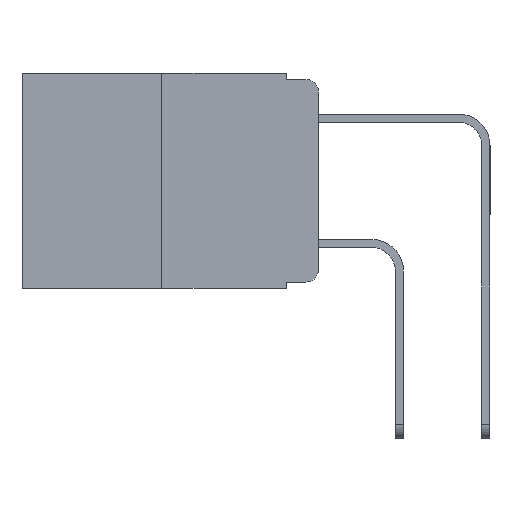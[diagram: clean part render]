
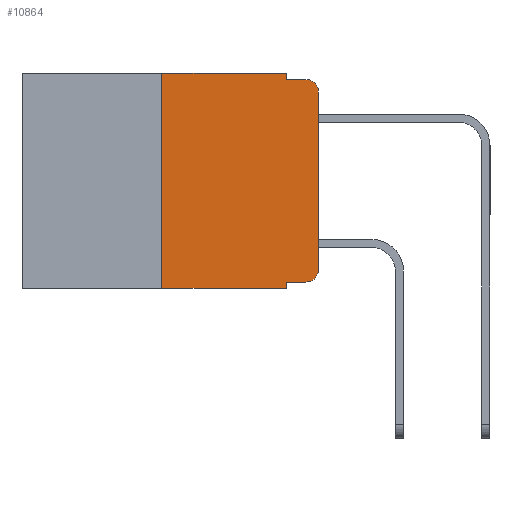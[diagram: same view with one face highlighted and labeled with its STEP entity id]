
A CAD part, left-side view. The second image highlights one B-rep face of the part: STEP entity #10864.
In plain terms, the highlighted planar face has unit normal (-1, 0, 0).
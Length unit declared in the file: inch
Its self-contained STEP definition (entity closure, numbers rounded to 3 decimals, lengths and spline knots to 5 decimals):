
#480 = CARTESIAN_POINT ( 'NONE',  ( 0., 0.051, 0. ) ) ;
#530 = LINE ( 'NONE', #8415, #14699 ) ;
#1100 = DIRECTION ( 'NONE',  ( 0., -1., 0. ) ) ;
#1102 = CIRCLE ( 'NONE', #14284, 0.02 ) ;
#1296 = CARTESIAN_POINT ( 'NONE',  ( 0., 0., 0. ) ) ;
#1386 = VERTEX_POINT ( 'NONE', #8026 ) ;
#1832 = DIRECTION ( 'NONE',  ( -1., 0., 0. ) ) ;
#1882 = DIRECTION ( 'NONE',  ( 0., 0., -1. ) ) ;
#2090 = PLANE ( 'NONE',  #13053 ) ;
#2598 = DIRECTION ( 'NONE',  ( 0., -1., 0. ) ) ;
#2621 = VERTEX_POINT ( 'NONE', #9906 ) ;
#2766 = CARTESIAN_POINT ( 'NONE',  ( 0., 0., -0.313 ) ) ;
#3625 = CARTESIAN_POINT ( 'NONE',  ( 0., 0.473, 0. ) ) ;
#4057 = EDGE_LOOP ( 'NONE', ( #8170, #14215, #16428, #11961, #13609, #15062, #17123, #9033, #10760, #8402 ) ) ;
#4405 = VERTEX_POINT ( 'NONE', #8011 ) ;
#4458 = LINE ( 'NONE', #8059, #11484 ) ;
#4533 = DIRECTION ( 'NONE',  ( 0., 0., 1. ) ) ;
#4945 = DIRECTION ( 'NONE',  ( 0., 0., -1. ) ) ;
#5331 = VERTEX_POINT ( 'NONE', #17863 ) ;
#5490 = CARTESIAN_POINT ( 'NONE',  ( 0., 0.473, 0. ) ) ;
#5586 = EDGE_CURVE ( 'NONE', #4405, #9103, #1102, .T. ) ;
#6154 = LINE ( 'NONE', #11848, #13022 ) ;
#6484 = FACE_OUTER_BOUND ( 'NONE', #4057, .T. ) ;
#6548 = DIRECTION ( 'NONE',  ( 0., 0., -1. ) ) ;
#6557 = EDGE_CURVE ( 'NONE', #1386, #4405, #530, .T. ) ;
#7284 = CARTESIAN_POINT ( 'NONE',  ( 0., 0., -0.03 ) ) ;
#7324 = CARTESIAN_POINT ( 'NONE',  ( 0., 0.051, -0.01 ) ) ;
#7460 = CARTESIAN_POINT ( 'NONE',  ( 0., 0.02, -0.03 ) ) ;
#7497 = EDGE_CURVE ( 'NONE', #1386, #2621, #6154, .T. ) ;
#7759 = VERTEX_POINT ( 'NONE', #15169 ) ;
#8011 = CARTESIAN_POINT ( 'NONE',  ( 0., 0.02, -0.333 ) ) ;
#8026 = CARTESIAN_POINT ( 'NONE',  ( 0., 0.051, -0.333 ) ) ;
#8059 = CARTESIAN_POINT ( 'NONE',  ( 0., 0.051, -0.01 ) ) ;
#8170 = ORIENTED_EDGE ( 'NONE', *, *, #12098, .T. ) ;
#8171 = VECTOR ( 'NONE', #10193, 39.37008 ) ;
#8244 = CIRCLE ( 'NONE', #10957, 0.02 ) ;
#8402 = ORIENTED_EDGE ( 'NONE', *, *, #5586, .T. ) ;
#8415 = CARTESIAN_POINT ( 'NONE',  ( 0., 0.051, -0.333 ) ) ;
#8440 = EDGE_CURVE ( 'NONE', #9852, #5331, #8981, .T. ) ;
#8602 = LINE ( 'NONE', #8787, #8171 ) ;
#8787 = CARTESIAN_POINT ( 'NONE',  ( 0., 0.473, -0.343 ) ) ;
#8847 = DIRECTION ( 'NONE',  ( 0., 0., -1. ) ) ;
#8926 = VERTEX_POINT ( 'NONE', #480 ) ;
#8981 = LINE ( 'NONE', #10157, #12197 ) ;
#9033 = ORIENTED_EDGE ( 'NONE', *, *, #7497, .F. ) ;
#9097 = CARTESIAN_POINT ( 'NONE',  ( 0., 0.051, 0. ) ) ;
#9103 = VERTEX_POINT ( 'NONE', #2766 ) ;
#9157 = VECTOR ( 'NONE', #1882, 39.37008 ) ;
#9165 = VERTEX_POINT ( 'NONE', #7284 ) ;
#9296 = VECTOR ( 'NONE', #11240, 39.37008 ) ;
#9353 = EDGE_CURVE ( 'NONE', #8926, #9755, #9608, .T. ) ;
#9608 = LINE ( 'NONE', #9097, #9157 ) ;
#9755 = VERTEX_POINT ( 'NONE', #7324 ) ;
#9852 = VERTEX_POINT ( 'NONE', #16800 ) ;
#9906 = CARTESIAN_POINT ( 'NONE',  ( 0., 0.051, -0.343 ) ) ;
#9946 = VECTOR ( 'NONE', #2598, 39.37008 ) ;
#10157 = CARTESIAN_POINT ( 'NONE',  ( 0., 0.25, 0. ) ) ;
#10193 = DIRECTION ( 'NONE',  ( 0., -1., 0. ) ) ;
#10279 = EDGE_CURVE ( 'NONE', #9755, #7759, #4458, .T. ) ;
#10437 = CARTESIAN_POINT ( 'NONE',  ( 0., 0.02, -0.313 ) ) ;
#10760 = ORIENTED_EDGE ( 'NONE', *, *, #6557, .T. ) ;
#10864 = ADVANCED_FACE ( 'NONE', ( #6484 ), #2090, .F. ) ;
#10957 = AXIS2_PLACEMENT_3D ( 'NONE', #7460, #16825, #8847 ) ;
#11209 = EDGE_CURVE ( 'NONE', #9165, #7759, #8244, .T. ) ;
#11240 = DIRECTION ( 'NONE',  ( 0., 0., 1. ) ) ;
#11484 = VECTOR ( 'NONE', #17371, 39.37008 ) ;
#11811 = DIRECTION ( 'NONE',  ( 0., 0., -1. ) ) ;
#11848 = CARTESIAN_POINT ( 'NONE',  ( 0., 0.051, 0. ) ) ;
#11961 = ORIENTED_EDGE ( 'NONE', *, *, #9353, .F. ) ;
#12075 = LINE ( 'NONE', #1296, #9296 ) ;
#12098 = EDGE_CURVE ( 'NONE', #9103, #9165, #12075, .T. ) ;
#12197 = VECTOR ( 'NONE', #4533, 39.37008 ) ;
#13022 = VECTOR ( 'NONE', #4945, 39.37008 ) ;
#13053 = AXIS2_PLACEMENT_3D ( 'NONE', #3625, #14660, #6548 ) ;
#13609 = ORIENTED_EDGE ( 'NONE', *, *, #15982, .F. ) ;
#13758 = EDGE_CURVE ( 'NONE', #9852, #2621, #8602, .T. ) ;
#13915 = LINE ( 'NONE', #5490, #9946 ) ;
#14215 = ORIENTED_EDGE ( 'NONE', *, *, #11209, .T. ) ;
#14284 = AXIS2_PLACEMENT_3D ( 'NONE', #10437, #1832, #11811 ) ;
#14660 = DIRECTION ( 'NONE',  ( 1., 0., 0. ) ) ;
#14699 = VECTOR ( 'NONE', #1100, 39.37008 ) ;
#15062 = ORIENTED_EDGE ( 'NONE', *, *, #8440, .F. ) ;
#15169 = CARTESIAN_POINT ( 'NONE',  ( 0., 0.02, -0.01 ) ) ;
#15982 = EDGE_CURVE ( 'NONE', #5331, #8926, #13915, .T. ) ;
#16428 = ORIENTED_EDGE ( 'NONE', *, *, #10279, .F. ) ;
#16800 = CARTESIAN_POINT ( 'NONE',  ( 0., 0.25, -0.343 ) ) ;
#16825 = DIRECTION ( 'NONE',  ( -1., 0., 0. ) ) ;
#17123 = ORIENTED_EDGE ( 'NONE', *, *, #13758, .T. ) ;
#17371 = DIRECTION ( 'NONE',  ( 0., -1., 0. ) ) ;
#17863 = CARTESIAN_POINT ( 'NONE',  ( 0., 0.25, 0. ) ) ;
